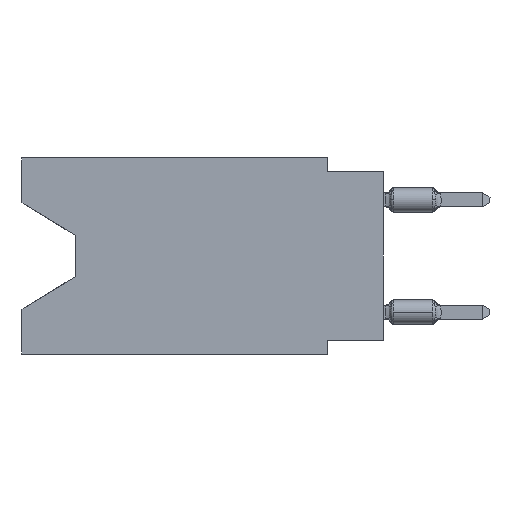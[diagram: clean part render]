
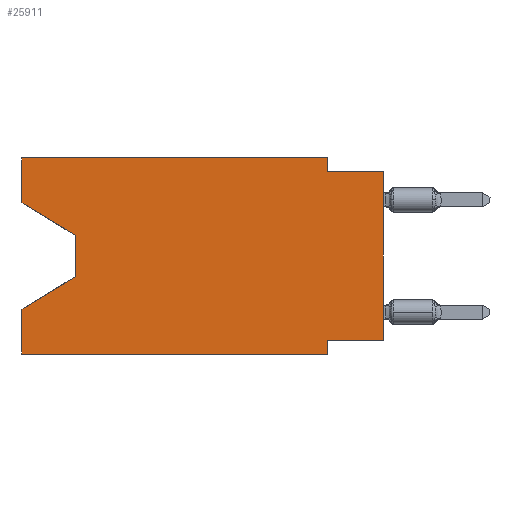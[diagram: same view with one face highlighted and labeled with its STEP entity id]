
A CAD part, left-side view. The second image highlights one B-rep face of the part: STEP entity #25911.
In plain terms, the highlighted planar face has unit normal (-1, 0, 0).
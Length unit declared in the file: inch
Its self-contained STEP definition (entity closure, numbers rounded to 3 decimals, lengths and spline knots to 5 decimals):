
#192 = PLANE ( 'NONE',  #21239 ) ;
#437 = DIRECTION ( 'NONE',  ( 0., 0., 1. ) ) ;
#513 = CARTESIAN_POINT ( 'NONE',  ( 0., 0.645, -0.08025 ) ) ;
#682 = VERTEX_POINT ( 'NONE', #14579 ) ;
#1464 = LINE ( 'NONE', #10116, #10763 ) ;
#2206 = DIRECTION ( 'NONE',  ( 0., 0., -1. ) ) ;
#2356 = EDGE_CURVE ( 'NONE', #15595, #9072, #25685, .T. ) ;
#2614 = ORIENTED_EDGE ( 'NONE', *, *, #2356, .T. ) ;
#2708 = CARTESIAN_POINT ( 'NONE',  ( 0., 0.55, -0.138 ) ) ;
#2780 = ORIENTED_EDGE ( 'NONE', *, *, #10235, .F. ) ;
#3147 = CARTESIAN_POINT ( 'NONE',  ( 0., 0.55, -0.212 ) ) ;
#3284 = DIRECTION ( 'NONE',  ( 0., 0.855, -0.519 ) ) ;
#4141 = DIRECTION ( 'NONE',  ( 0., 0., -1. ) ) ;
#4326 = CARTESIAN_POINT ( 'NONE',  ( 0., 0.645, 0. ) ) ;
#4497 = ORIENTED_EDGE ( 'NONE', *, *, #17681, .T. ) ;
#4540 = CARTESIAN_POINT ( 'NONE',  ( 0., 0.55, -0.138 ) ) ;
#4867 = EDGE_CURVE ( 'NONE', #18135, #18393, #8493, .T. ) ;
#4932 = LINE ( 'NONE', #17270, #25745 ) ;
#5599 = DIRECTION ( 'NONE',  ( 0., -1., 0. ) ) ;
#5739 = VERTEX_POINT ( 'NONE', #21210 ) ;
#6009 = LINE ( 'NONE', #16348, #19361 ) ;
#6182 = CARTESIAN_POINT ( 'NONE',  ( 0., 0.645, 0. ) ) ;
#6289 = LINE ( 'NONE', #14490, #15365 ) ;
#6636 = DIRECTION ( 'NONE',  ( 0., -0.855, -0.519 ) ) ;
#6643 = VECTOR ( 'NONE', #5599, 39.37008 ) ;
#6732 = VERTEX_POINT ( 'NONE', #9218 ) ;
#6814 = VERTEX_POINT ( 'NONE', #11584 ) ;
#6949 = EDGE_CURVE ( 'NONE', #24378, #19617, #6009, .T. ) ;
#7200 = ORIENTED_EDGE ( 'NONE', *, *, #13870, .T. ) ;
#7289 = ORIENTED_EDGE ( 'NONE', *, *, #18832, .F. ) ;
#7510 = VERTEX_POINT ( 'NONE', #7532 ) ;
#7532 = CARTESIAN_POINT ( 'NONE',  ( 0., 0.1, -0.35 ) ) ;
#7958 = CARTESIAN_POINT ( 'NONE',  ( 0., 0.1, -0.025 ) ) ;
#7974 = CARTESIAN_POINT ( 'NONE',  ( 0., 0., -0.325 ) ) ;
#8129 = DIRECTION ( 'NONE',  ( 0., 0., -1. ) ) ;
#8493 = LINE ( 'NONE', #17085, #22706 ) ;
#8736 = ORIENTED_EDGE ( 'NONE', *, *, #15033, .F. ) ;
#9011 = LINE ( 'NONE', #3147, #13104 ) ;
#9072 = VERTEX_POINT ( 'NONE', #15182 ) ;
#9218 = CARTESIAN_POINT ( 'NONE',  ( 0., 0.645, -0.35 ) ) ;
#9294 = ORIENTED_EDGE ( 'NONE', *, *, #25139, .F. ) ;
#10054 = DIRECTION ( 'NONE',  ( 1., 0., 0. ) ) ;
#10116 = CARTESIAN_POINT ( 'NONE',  ( 0., 0.645, 0. ) ) ;
#10235 = EDGE_CURVE ( 'NONE', #682, #7510, #6289, .T. ) ;
#10478 = EDGE_CURVE ( 'NONE', #6732, #5739, #1464, .T. ) ;
#10559 = LINE ( 'NONE', #6182, #22929 ) ;
#10575 = VECTOR ( 'NONE', #14943, 39.37008 ) ;
#10763 = VECTOR ( 'NONE', #24053, 39.37008 ) ;
#11584 = CARTESIAN_POINT ( 'NONE',  ( 0., 0.645, 0. ) ) ;
#11599 = LINE ( 'NONE', #17702, #17722 ) ;
#13104 = VECTOR ( 'NONE', #3284, 39.37008 ) ;
#13506 = VERTEX_POINT ( 'NONE', #24872 ) ;
#13589 = CARTESIAN_POINT ( 'NONE',  ( 0., 0., 0. ) ) ;
#13870 = EDGE_CURVE ( 'NONE', #18393, #13506, #24723, .T. ) ;
#14490 = CARTESIAN_POINT ( 'NONE',  ( 0., 0.1, -0.35 ) ) ;
#14579 = CARTESIAN_POINT ( 'NONE',  ( 0., 0.1, -0.325 ) ) ;
#14943 = DIRECTION ( 'NONE',  ( 0., 0., 1. ) ) ;
#15033 = EDGE_CURVE ( 'NONE', #6814, #24378, #23806, .T. ) ;
#15173 = ORIENTED_EDGE ( 'NONE', *, *, #21065, .F. ) ;
#15182 = CARTESIAN_POINT ( 'NONE',  ( 0., 0., -0.025 ) ) ;
#15222 = CARTESIAN_POINT ( 'NONE',  ( 0., 0.1, 0. ) ) ;
#15365 = VECTOR ( 'NONE', #18886, 39.37008 ) ;
#15595 = VERTEX_POINT ( 'NONE', #7974 ) ;
#16348 = CARTESIAN_POINT ( 'NONE',  ( 0., 0.1, 0. ) ) ;
#16494 = LINE ( 'NONE', #18362, #19403 ) ;
#17085 = CARTESIAN_POINT ( 'NONE',  ( 0., 0.645, -0.08025 ) ) ;
#17270 = CARTESIAN_POINT ( 'NONE',  ( 0., 0.645, -0.35 ) ) ;
#17396 = EDGE_LOOP ( 'NONE', ( #20310, #7200, #18323, #24150, #4497, #2780, #7289, #2614, #15173, #24011, #8736, #9294 ) ) ;
#17681 = EDGE_CURVE ( 'NONE', #6732, #7510, #4932, .T. ) ;
#17702 = CARTESIAN_POINT ( 'NONE',  ( 0., 0., -0.025 ) ) ;
#17722 = VECTOR ( 'NONE', #19830, 39.37008 ) ;
#18135 = VERTEX_POINT ( 'NONE', #513 ) ;
#18323 = ORIENTED_EDGE ( 'NONE', *, *, #22165, .T. ) ;
#18362 = CARTESIAN_POINT ( 'NONE',  ( 0., 0., -0.325 ) ) ;
#18393 = VERTEX_POINT ( 'NONE', #2708 ) ;
#18401 = FACE_OUTER_BOUND ( 'NONE', #17396, .T. ) ;
#18832 = EDGE_CURVE ( 'NONE', #15595, #682, #16494, .T. ) ;
#18886 = DIRECTION ( 'NONE',  ( 0., 0., -1. ) ) ;
#19361 = VECTOR ( 'NONE', #4141, 39.37008 ) ;
#19403 = VECTOR ( 'NONE', #22226, 39.37008 ) ;
#19617 = VERTEX_POINT ( 'NONE', #7958 ) ;
#19830 = DIRECTION ( 'NONE',  ( 0., -1., 0. ) ) ;
#20310 = ORIENTED_EDGE ( 'NONE', *, *, #4867, .T. ) ;
#21065 = EDGE_CURVE ( 'NONE', #19617, #9072, #11599, .T. ) ;
#21210 = CARTESIAN_POINT ( 'NONE',  ( 0., 0.645, -0.26975 ) ) ;
#21239 = AXIS2_PLACEMENT_3D ( 'NONE', #4326, #10054, #2206 ) ;
#22165 = EDGE_CURVE ( 'NONE', #13506, #5739, #9011, .T. ) ;
#22226 = DIRECTION ( 'NONE',  ( 0., 1., 0. ) ) ;
#22706 = VECTOR ( 'NONE', #6636, 39.37008 ) ;
#22929 = VECTOR ( 'NONE', #437, 39.37008 ) ;
#23806 = LINE ( 'NONE', #23928, #6643 ) ;
#23928 = CARTESIAN_POINT ( 'NONE',  ( 0., 0.645, 0. ) ) ;
#24011 = ORIENTED_EDGE ( 'NONE', *, *, #6949, .F. ) ;
#24053 = DIRECTION ( 'NONE',  ( 0., 0., 1. ) ) ;
#24150 = ORIENTED_EDGE ( 'NONE', *, *, #10478, .F. ) ;
#24378 = VERTEX_POINT ( 'NONE', #15222 ) ;
#24723 = LINE ( 'NONE', #4540, #26064 ) ;
#24872 = CARTESIAN_POINT ( 'NONE',  ( 0., 0.55, -0.212 ) ) ;
#25139 = EDGE_CURVE ( 'NONE', #18135, #6814, #10559, .T. ) ;
#25249 = DIRECTION ( 'NONE',  ( 0., -1., 0. ) ) ;
#25685 = LINE ( 'NONE', #13589, #10575 ) ;
#25745 = VECTOR ( 'NONE', #25249, 39.37008 ) ;
#25911 = ADVANCED_FACE ( 'NONE', ( #18401 ), #192, .F. ) ;
#26064 = VECTOR ( 'NONE', #8129, 39.37008 ) ;
